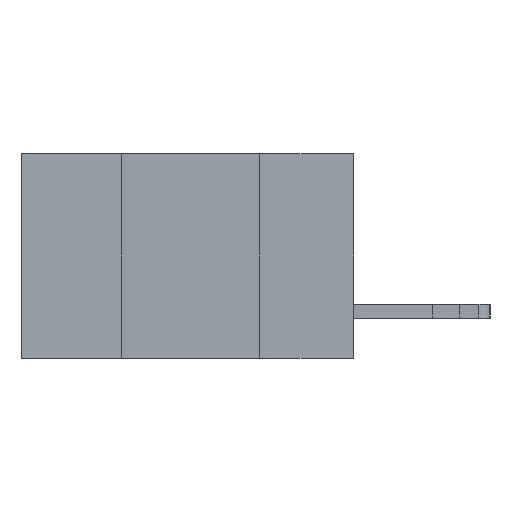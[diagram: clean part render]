
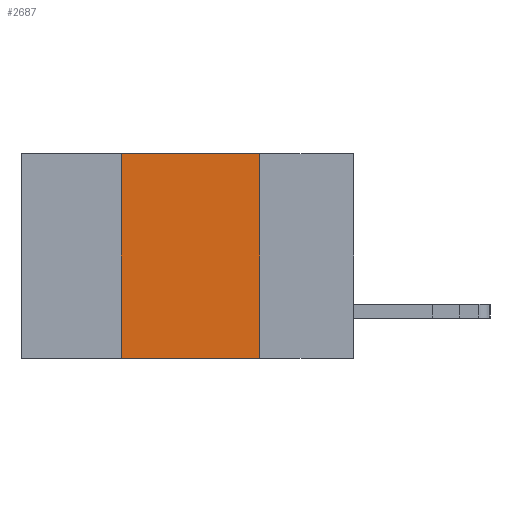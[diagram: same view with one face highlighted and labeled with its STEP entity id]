
A CAD part, left-side view. The second image highlights one B-rep face of the part: STEP entity #2687.
In plain terms, the highlighted planar face has unit normal (-1, 0, 0).
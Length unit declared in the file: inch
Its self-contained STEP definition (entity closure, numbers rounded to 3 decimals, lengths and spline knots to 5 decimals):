
#319 = ORIENTED_EDGE ( 'NONE', *, *, #8884, .F. ) ;
#523 = PLANE ( 'NONE',  #8473 ) ;
#682 = CARTESIAN_POINT ( 'NONE',  ( 0., 0.6, 0. ) ) ;
#1420 = VECTOR ( 'NONE', #4170, 39.37008 ) ;
#1807 = DIRECTION ( 'NONE',  ( 0., 0., -1. ) ) ;
#1870 = LINE ( 'NONE', #11895, #1420 ) ;
#2687 = ADVANCED_FACE ( 'NONE', ( #5400 ), #523, .F. ) ;
#3205 = ORIENTED_EDGE ( 'NONE', *, *, #13838, .F. ) ;
#3359 = VECTOR ( 'NONE', #11851, 39.37008 ) ;
#4024 = CARTESIAN_POINT ( 'NONE',  ( 0., 0.17, 0. ) ) ;
#4169 = DIRECTION ( 'NONE',  ( 0., 0., 1. ) ) ;
#4170 = DIRECTION ( 'NONE',  ( 0., -1., 0. ) ) ;
#4395 = DIRECTION ( 'NONE',  ( 0., 0., -1. ) ) ;
#5400 = FACE_OUTER_BOUND ( 'NONE', #9798, .T. ) ;
#5672 = LINE ( 'NONE', #12897, #3359 ) ;
#7507 = LINE ( 'NONE', #4024, #9698 ) ;
#7838 = VERTEX_POINT ( 'NONE', #10373 ) ;
#7891 = LINE ( 'NONE', #9117, #12537 ) ;
#8103 = ORIENTED_EDGE ( 'NONE', *, *, #13003, .F. ) ;
#8473 = AXIS2_PLACEMENT_3D ( 'NONE', #682, #15553, #4395 ) ;
#8884 = EDGE_CURVE ( 'NONE', #9206, #10899, #1870, .T. ) ;
#9117 = CARTESIAN_POINT ( 'NONE',  ( 0., 0.42, 0. ) ) ;
#9206 = VERTEX_POINT ( 'NONE', #16203 ) ;
#9698 = VECTOR ( 'NONE', #1807, 39.37008 ) ;
#9798 = EDGE_LOOP ( 'NONE', ( #3205, #319, #8103, #13132 ) ) ;
#10373 = CARTESIAN_POINT ( 'NONE',  ( 0., 0.42, -0.37 ) ) ;
#10899 = VERTEX_POINT ( 'NONE', #13509 ) ;
#11485 = EDGE_CURVE ( 'NONE', #7838, #14230, #5672, .T. ) ;
#11851 = DIRECTION ( 'NONE',  ( 0., -1., 0. ) ) ;
#11895 = CARTESIAN_POINT ( 'NONE',  ( 0., 0.6, 0. ) ) ;
#12537 = VECTOR ( 'NONE', #4169, 39.37008 ) ;
#12897 = CARTESIAN_POINT ( 'NONE',  ( 0., 0.6, -0.37 ) ) ;
#13003 = EDGE_CURVE ( 'NONE', #7838, #9206, #7891, .T. ) ;
#13132 = ORIENTED_EDGE ( 'NONE', *, *, #11485, .T. ) ;
#13509 = CARTESIAN_POINT ( 'NONE',  ( 0., 0.17, 0. ) ) ;
#13838 = EDGE_CURVE ( 'NONE', #10899, #14230, #7507, .T. ) ;
#14183 = CARTESIAN_POINT ( 'NONE',  ( 0., 0.17, -0.37 ) ) ;
#14230 = VERTEX_POINT ( 'NONE', #14183 ) ;
#15553 = DIRECTION ( 'NONE',  ( 1., 0., 0. ) ) ;
#16203 = CARTESIAN_POINT ( 'NONE',  ( 0., 0.42, 0. ) ) ;
